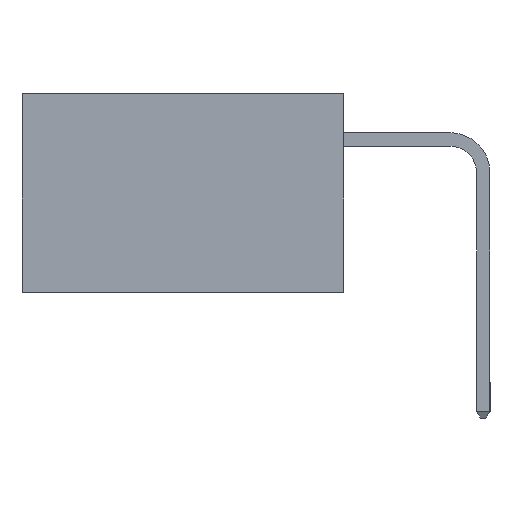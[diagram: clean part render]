
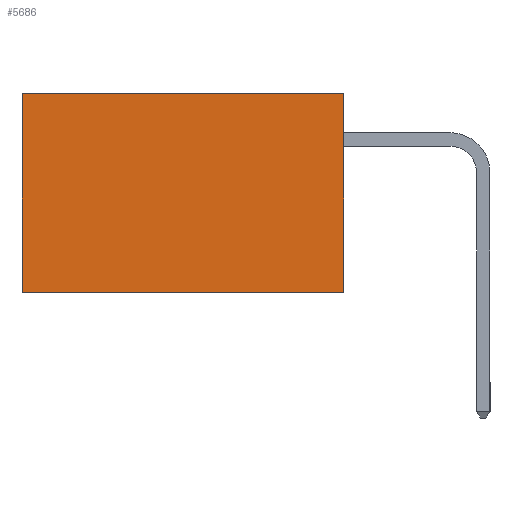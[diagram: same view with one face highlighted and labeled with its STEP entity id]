
A CAD part, left-side view. The second image highlights one B-rep face of the part: STEP entity #5686.
In plain terms, the highlighted planar face has unit normal (-1, 0, 0).
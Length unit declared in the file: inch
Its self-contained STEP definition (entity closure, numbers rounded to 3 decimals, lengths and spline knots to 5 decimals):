
#488 = DIRECTION ( 'NONE',  ( 0., 1., 0. ) ) ;
#630 = CARTESIAN_POINT ( 'NONE',  ( 0.298, 0., 0. ) ) ;
#876 = DIRECTION ( 'NONE',  ( 0., 1., 0. ) ) ;
#976 = VECTOR ( 'NONE', #488, 39.37008 ) ;
#1317 = CARTESIAN_POINT ( 'NONE',  ( 0.298, 0.6, 0. ) ) ;
#1617 = VERTEX_POINT ( 'NONE', #630 ) ;
#1958 = ORIENTED_EDGE ( 'NONE', *, *, #8834, .T. ) ;
#2282 = VERTEX_POINT ( 'NONE', #9849 ) ;
#2926 = VECTOR ( 'NONE', #876, 39.37008 ) ;
#2998 = CARTESIAN_POINT ( 'NONE',  ( 0.298, 0.6, -0.37 ) ) ;
#3180 = VERTEX_POINT ( 'NONE', #14461 ) ;
#3614 = EDGE_CURVE ( 'NONE', #1617, #2282, #4643, .T. ) ;
#4389 = AXIS2_PLACEMENT_3D ( 'NONE', #12822, #9177, #9035 ) ;
#4392 = ORIENTED_EDGE ( 'NONE', *, *, #4462, .F. ) ;
#4462 = EDGE_CURVE ( 'NONE', #2282, #8330, #6119, .T. ) ;
#4643 = LINE ( 'NONE', #7677, #10288 ) ;
#4838 = ORIENTED_EDGE ( 'NONE', *, *, #3614, .F. ) ;
#4898 = EDGE_CURVE ( 'NONE', #1617, #3180, #7410, .T. ) ;
#5097 = EDGE_LOOP ( 'NONE', ( #1958, #4392, #4838, #5103 ) ) ;
#5103 = ORIENTED_EDGE ( 'NONE', *, *, #4898, .T. ) ;
#5686 = ADVANCED_FACE ( 'NONE', ( #12879 ), #10349, .F. ) ;
#6119 = LINE ( 'NONE', #8095, #2926 ) ;
#7410 = LINE ( 'NONE', #7812, #976 ) ;
#7677 = CARTESIAN_POINT ( 'NONE',  ( 0.298, 0., 0. ) ) ;
#7812 = CARTESIAN_POINT ( 'NONE',  ( 0.298, 0., 0. ) ) ;
#8095 = CARTESIAN_POINT ( 'NONE',  ( 0.298, 0., -0.37 ) ) ;
#8330 = VERTEX_POINT ( 'NONE', #2998 ) ;
#8834 = EDGE_CURVE ( 'NONE', #3180, #8330, #11278, .T. ) ;
#9035 = DIRECTION ( 'NONE',  ( 0., 0., -1. ) ) ;
#9177 = DIRECTION ( 'NONE',  ( 1., 0., 0. ) ) ;
#9758 = VECTOR ( 'NONE', #9815, 39.37008 ) ;
#9815 = DIRECTION ( 'NONE',  ( 0., 0., -1. ) ) ;
#9849 = CARTESIAN_POINT ( 'NONE',  ( 0.298, 0., -0.37 ) ) ;
#10148 = DIRECTION ( 'NONE',  ( 0., 0., -1. ) ) ;
#10288 = VECTOR ( 'NONE', #10148, 39.37008 ) ;
#10349 = PLANE ( 'NONE',  #4389 ) ;
#11278 = LINE ( 'NONE', #1317, #9758 ) ;
#12822 = CARTESIAN_POINT ( 'NONE',  ( 0.298, 0., 0. ) ) ;
#12879 = FACE_OUTER_BOUND ( 'NONE', #5097, .T. ) ;
#14461 = CARTESIAN_POINT ( 'NONE',  ( 0.298, 0.6, 0. ) ) ;
